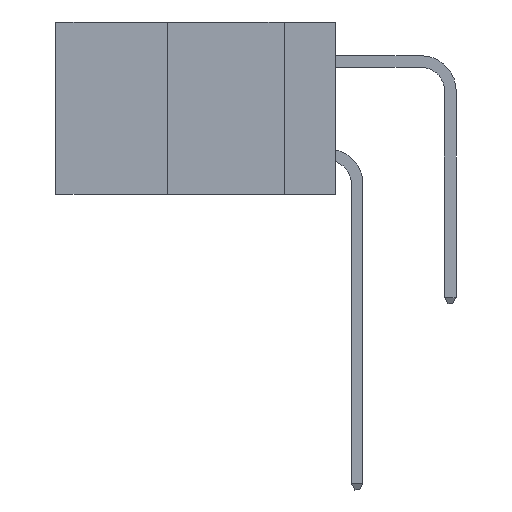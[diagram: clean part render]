
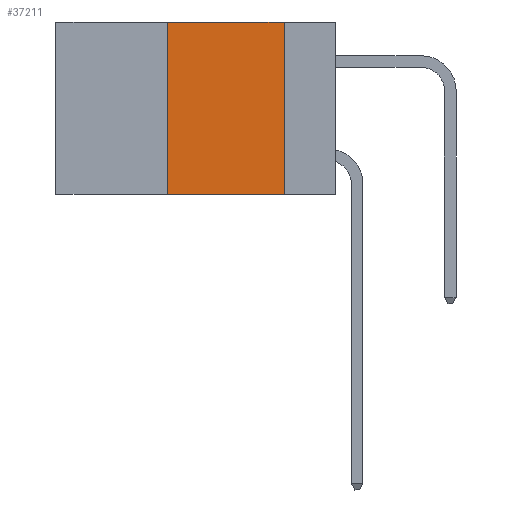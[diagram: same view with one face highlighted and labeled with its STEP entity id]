
A CAD part, left-side view. The second image highlights one B-rep face of the part: STEP entity #37211.
In plain terms, the highlighted planar face has unit normal (-1, 0, 0).
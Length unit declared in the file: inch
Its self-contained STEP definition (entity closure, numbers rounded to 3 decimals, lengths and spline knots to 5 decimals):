
#601 = VECTOR ( 'NONE', #31976, 39.37008 ) ;
#671 = VERTEX_POINT ( 'NONE', #8966 ) ;
#1709 = VECTOR ( 'NONE', #30127, 39.37008 ) ;
#2355 = PLANE ( 'NONE',  #7357 ) ;
#4050 = EDGE_LOOP ( 'NONE', ( #39002, #10873, #11115, #19227 ) ) ;
#5511 = DIRECTION ( 'NONE',  ( 1., 0., 0. ) ) ;
#7357 = AXIS2_PLACEMENT_3D ( 'NONE', #24392, #5511, #27478 ) ;
#8966 = CARTESIAN_POINT ( 'NONE',  ( 0., 0.36, 0. ) ) ;
#9075 = LINE ( 'NONE', #38082, #601 ) ;
#10873 = ORIENTED_EDGE ( 'NONE', *, *, #16675, .F. ) ;
#11115 = ORIENTED_EDGE ( 'NONE', *, *, #38396, .F. ) ;
#14281 = LINE ( 'NONE', #19043, #38086 ) ;
#14654 = CARTESIAN_POINT ( 'NONE',  ( 0., 0.6, 0. ) ) ;
#15240 = EDGE_CURVE ( 'NONE', #27272, #32801, #25462, .T. ) ;
#16434 = CARTESIAN_POINT ( 'NONE',  ( 0., 0.11, 0. ) ) ;
#16675 = EDGE_CURVE ( 'NONE', #671, #24522, #19549, .T. ) ;
#19043 = CARTESIAN_POINT ( 'NONE',  ( 0., 0.36, 0. ) ) ;
#19205 = CARTESIAN_POINT ( 'NONE',  ( 0., 0.36, -0.37 ) ) ;
#19227 = ORIENTED_EDGE ( 'NONE', *, *, #15240, .T. ) ;
#19549 = LINE ( 'NONE', #14654, #1709 ) ;
#22185 = DIRECTION ( 'NONE',  ( 0., 0., 1. ) ) ;
#24392 = CARTESIAN_POINT ( 'NONE',  ( 0., 0.6, 0. ) ) ;
#24522 = VERTEX_POINT ( 'NONE', #16434 ) ;
#25172 = EDGE_CURVE ( 'NONE', #24522, #32801, #9075, .T. ) ;
#25462 = LINE ( 'NONE', #35962, #28835 ) ;
#27272 = VERTEX_POINT ( 'NONE', #19205 ) ;
#27478 = DIRECTION ( 'NONE',  ( 0., 0., -1. ) ) ;
#28835 = VECTOR ( 'NONE', #39030, 39.37008 ) ;
#30127 = DIRECTION ( 'NONE',  ( 0., -1., 0. ) ) ;
#31976 = DIRECTION ( 'NONE',  ( 0., 0., -1. ) ) ;
#32801 = VERTEX_POINT ( 'NONE', #38265 ) ;
#35962 = CARTESIAN_POINT ( 'NONE',  ( 0., 0.6, -0.37 ) ) ;
#36297 = FACE_OUTER_BOUND ( 'NONE', #4050, .T. ) ;
#37211 = ADVANCED_FACE ( 'NONE', ( #36297 ), #2355, .F. ) ;
#38082 = CARTESIAN_POINT ( 'NONE',  ( 0., 0.11, 0. ) ) ;
#38086 = VECTOR ( 'NONE', #22185, 39.37008 ) ;
#38265 = CARTESIAN_POINT ( 'NONE',  ( 0., 0.11, -0.37 ) ) ;
#38396 = EDGE_CURVE ( 'NONE', #27272, #671, #14281, .T. ) ;
#39002 = ORIENTED_EDGE ( 'NONE', *, *, #25172, .F. ) ;
#39030 = DIRECTION ( 'NONE',  ( 0., -1., 0. ) ) ;
